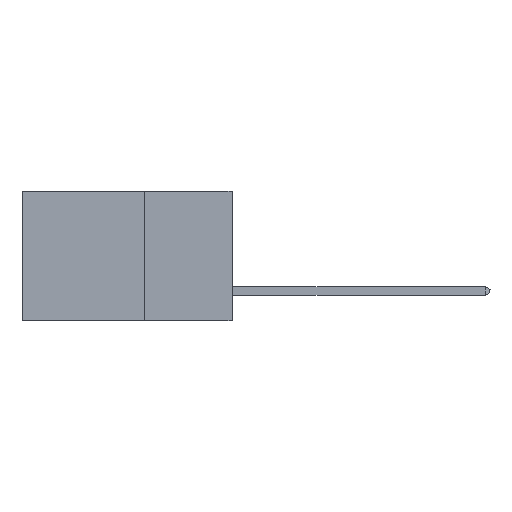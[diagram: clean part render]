
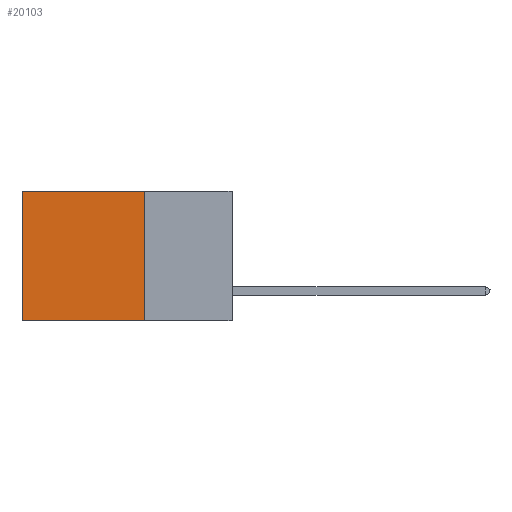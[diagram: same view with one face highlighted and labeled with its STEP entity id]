
A CAD part, left-side view. The second image highlights one B-rep face of the part: STEP entity #20103.
In plain terms, the highlighted planar face has unit normal (-1, 0, 0).
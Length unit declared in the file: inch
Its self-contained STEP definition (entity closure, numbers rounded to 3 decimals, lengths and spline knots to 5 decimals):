
#558 = DIRECTION ( 'NONE',  ( 0., 1., 0. ) ) ;
#1272 = DIRECTION ( 'NONE',  ( 0., 1., 0. ) ) ;
#1498 = EDGE_CURVE ( 'NONE', #5312, #18360, #4708, .T. ) ;
#2598 = DIRECTION ( 'NONE',  ( 0., 0., -1. ) ) ;
#3201 = ORIENTED_EDGE ( 'NONE', *, *, #22826, .F. ) ;
#4537 = VECTOR ( 'NONE', #1272, 39.37008 ) ;
#4708 = LINE ( 'NONE', #19333, #34993 ) ;
#5312 = VERTEX_POINT ( 'NONE', #19008 ) ;
#5665 = AXIS2_PLACEMENT_3D ( 'NONE', #6394, #10136, #2598 ) ;
#6394 = CARTESIAN_POINT ( 'NONE',  ( 0.2875, 0.25, 0. ) ) ;
#10136 = DIRECTION ( 'NONE',  ( 1., 0., 0. ) ) ;
#12065 = VECTOR ( 'NONE', #16579, 39.37008 ) ;
#12682 = VERTEX_POINT ( 'NONE', #34872 ) ;
#13675 = CARTESIAN_POINT ( 'NONE',  ( 0.2875, 0.6, 0. ) ) ;
#13684 = EDGE_CURVE ( 'NONE', #5312, #12682, #30544, .T. ) ;
#16579 = DIRECTION ( 'NONE',  ( 0., 0., -1. ) ) ;
#18360 = VERTEX_POINT ( 'NONE', #31412 ) ;
#18389 = VERTEX_POINT ( 'NONE', #32460 ) ;
#19008 = CARTESIAN_POINT ( 'NONE',  ( 0.2875, 0.25, 0. ) ) ;
#19333 = CARTESIAN_POINT ( 'NONE',  ( 0.2875, 0.25, 0. ) ) ;
#20103 = ADVANCED_FACE ( 'NONE', ( #36370 ), #20644, .F. ) ;
#20644 = PLANE ( 'NONE',  #5665 ) ;
#21524 = LINE ( 'NONE', #34877, #4537 ) ;
#22052 = LINE ( 'NONE', #13675, #12065 ) ;
#22826 = EDGE_CURVE ( 'NONE', #12682, #18389, #21524, .T. ) ;
#25099 = CARTESIAN_POINT ( 'NONE',  ( 0.2875, 0.25, 0. ) ) ;
#28443 = EDGE_CURVE ( 'NONE', #18360, #18389, #22052, .T. ) ;
#30544 = LINE ( 'NONE', #25099, #37552 ) ;
#31166 = ORIENTED_EDGE ( 'NONE', *, *, #28443, .T. ) ;
#31412 = CARTESIAN_POINT ( 'NONE',  ( 0.2875, 0.6, 0. ) ) ;
#32251 = DIRECTION ( 'NONE',  ( 0., 0., -1. ) ) ;
#32460 = CARTESIAN_POINT ( 'NONE',  ( 0.2875, 0.6, -0.37 ) ) ;
#34613 = ORIENTED_EDGE ( 'NONE', *, *, #13684, .F. ) ;
#34872 = CARTESIAN_POINT ( 'NONE',  ( 0.2875, 0.25, -0.37 ) ) ;
#34877 = CARTESIAN_POINT ( 'NONE',  ( 0.2875, 0.25, -0.37 ) ) ;
#34993 = VECTOR ( 'NONE', #558, 39.37008 ) ;
#36370 = FACE_OUTER_BOUND ( 'NONE', #41674, .T. ) ;
#37552 = VECTOR ( 'NONE', #32251, 39.37008 ) ;
#38579 = ORIENTED_EDGE ( 'NONE', *, *, #1498, .T. ) ;
#41674 = EDGE_LOOP ( 'NONE', ( #31166, #3201, #34613, #38579 ) ) ;
